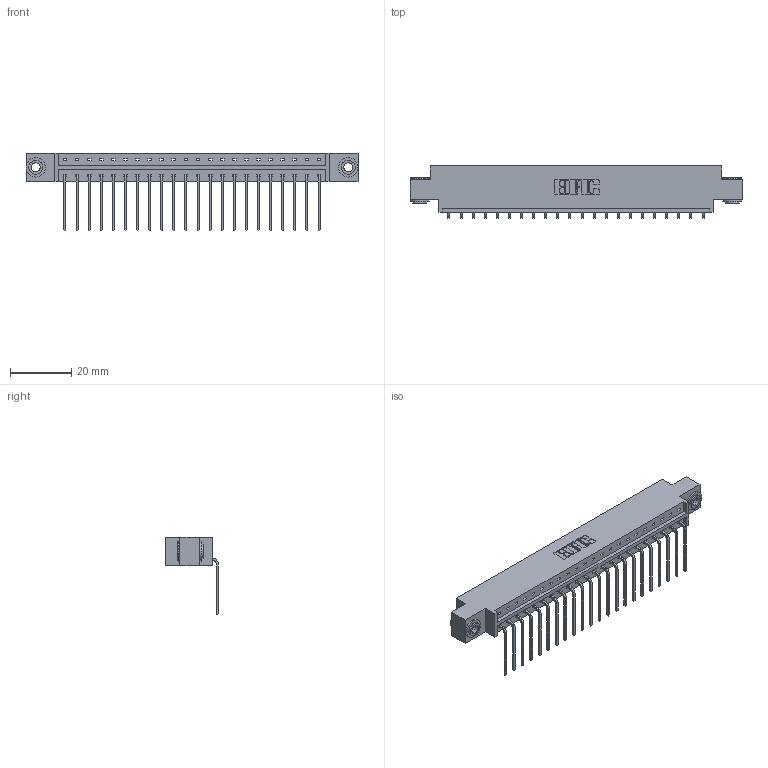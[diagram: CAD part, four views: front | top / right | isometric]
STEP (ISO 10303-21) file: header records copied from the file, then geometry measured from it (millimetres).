
FILE_DESCRIPTION (( 'STEP AP203' ), '1' );
FILE_NAME ('833-022-559-603.STEP', '2020-06-01T18:19:59', ( '' ), ( '' ), 'SwSTEP 2.0', 'SolidWorks 2020', '' );
FILE_SCHEMA (( 'CONFIG_CONTROL_DESIGN' ));
Length unit declared in the file: inch
Products named in the file (4): 833-022-559-603; 345-250-002_345-250-002-102; 345-292-001_558 559 Tail - 1; 833 Part_Offset - .156 Dia - TH
Assembly tree (25 placements, depth 2):
  833-022-559-603
    833 Part_Offset - .156 Dia - TH
    345-292-001_558 559 Tail - 1  x22
    345-250-002_345-250-002-102  x2
Bounding box: 108.71 x 17.09 x 25.53 mm (x, y, z)
Volume: 10632.4 mm3; surface area: 12248.2 mm2
Topology: 25 solids, 25 shells, 1476 faces, 4403 edges, 2902 vertices
Faces by surface type: plane 1052, cylinder 416, cone 8
Entity records: 16902 total; most frequent: CARTESIAN_POINT 2899, ORIENTED_EDGE 2850, DIRECTION 2519, EDGE_CURVE 1425, VECTOR 1273, LINE 1273, VERTEX_POINT 946, AXIS2_PLACEMENT_3D 623
